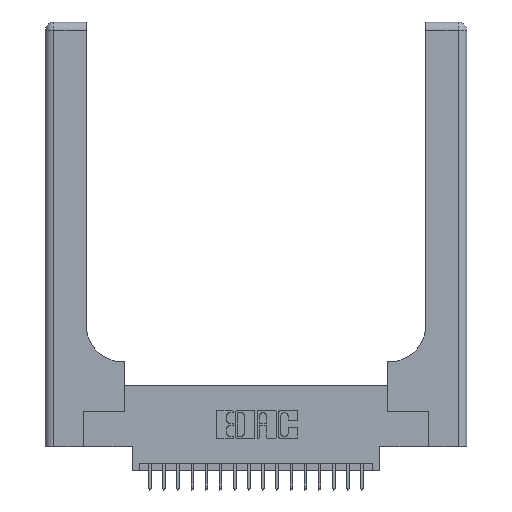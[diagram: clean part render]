
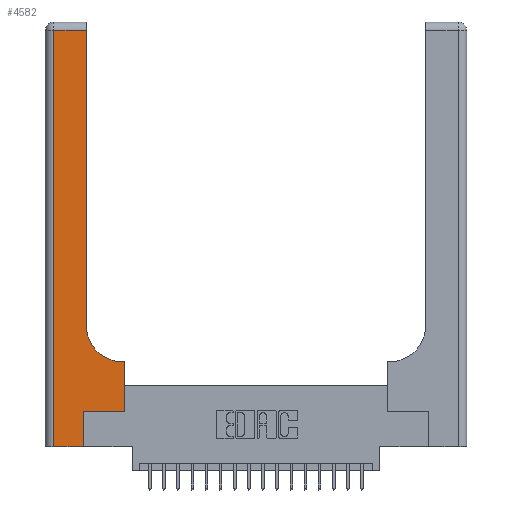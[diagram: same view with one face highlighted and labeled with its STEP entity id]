
A CAD part, top view. The second image highlights one B-rep face of the part: STEP entity #4582.
In plain terms, the highlighted planar face has unit normal (0, 0, 1).
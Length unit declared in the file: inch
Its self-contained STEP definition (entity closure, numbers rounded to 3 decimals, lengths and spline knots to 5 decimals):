
#65 = VECTOR ( 'NONE', #2025, 39.37008 ) ;
#373 = ORIENTED_EDGE ( 'NONE', *, *, #1104, .T. ) ;
#725 = LINE ( 'NONE', #10948, #19085 ) ;
#1032 = LINE ( 'NONE', #9504, #5738 ) ;
#1104 = EDGE_CURVE ( 'NONE', #9054, #12072, #725, .T. ) ;
#1222 = DIRECTION ( 'NONE',  ( 0., 1., 0. ) ) ;
#1312 = DIRECTION ( 'NONE',  ( 1., 0., 0. ) ) ;
#1569 = ORIENTED_EDGE ( 'NONE', *, *, #2822, .T. ) ;
#1586 = CARTESIAN_POINT ( 'NONE',  ( 0.2915, 0.85, 0.37 ) ) ;
#1832 = VECTOR ( 'NONE', #1312, 39.37008 ) ;
#2025 = DIRECTION ( 'NONE',  ( 0., 1., 0. ) ) ;
#2131 = CARTESIAN_POINT ( 'NONE',  ( 0.2915, 3., 0.37 ) ) ;
#2689 = ORIENTED_EDGE ( 'NONE', *, *, #15109, .T. ) ;
#2710 = ORIENTED_EDGE ( 'NONE', *, *, #3359, .T. ) ;
#2822 = EDGE_CURVE ( 'NONE', #18340, #11618, #16346, .T. ) ;
#2867 = LINE ( 'NONE', #9477, #3007 ) ;
#2895 = DIRECTION ( 'NONE',  ( 0., -1., 0. ) ) ;
#3000 = DIRECTION ( 'NONE',  ( -1., 0., 0. ) ) ;
#3007 = VECTOR ( 'NONE', #1222, 39.37008 ) ;
#3126 = PLANE ( 'NONE',  #5257 ) ;
#3159 = DIRECTION ( 'NONE',  ( 0., 0., -1. ) ) ;
#3212 = CARTESIAN_POINT ( 'NONE',  ( 0.2915, 0.6, 0.37 ) ) ;
#3359 = EDGE_CURVE ( 'NONE', #11618, #13096, #11821, .T. ) ;
#3872 = EDGE_CURVE ( 'NONE', #13096, #9054, #20190, .T. ) ;
#4400 = VECTOR ( 'NONE', #17076, 39.37008 ) ;
#4582 = ADVANCED_FACE ( 'NONE', ( #13520 ), #3126, .F. ) ;
#4727 = EDGE_LOOP ( 'NONE', ( #6545, #373, #9409, #11689, #12705, #2689, #13327, #1569, #2710 ) ) ;
#4884 = AXIS2_PLACEMENT_3D ( 'NONE', #16838, #3159, #9756 ) ;
#5224 = CARTESIAN_POINT ( 'NONE',  ( 0.5585, 0.25, 0.37 ) ) ;
#5257 = AXIS2_PLACEMENT_3D ( 'NONE', #11797, #18008, #20179 ) ;
#5450 = EDGE_CURVE ( 'NONE', #14862, #18210, #11525, .T. ) ;
#5738 = VECTOR ( 'NONE', #2895, 39.37008 ) ;
#6545 = ORIENTED_EDGE ( 'NONE', *, *, #3872, .T. ) ;
#7923 = CARTESIAN_POINT ( 'NONE',  ( 0.5585, 0.25, 0.37 ) ) ;
#8680 = VECTOR ( 'NONE', #3000, 39.37008 ) ;
#9054 = VERTEX_POINT ( 'NONE', #18430 ) ;
#9409 = ORIENTED_EDGE ( 'NONE', *, *, #19725, .T. ) ;
#9477 = CARTESIAN_POINT ( 'NONE',  ( 0.269, 0., 0.37 ) ) ;
#9504 = CARTESIAN_POINT ( 'NONE',  ( 0.06, 3., 0.37 ) ) ;
#9584 = DIRECTION ( 'NONE',  ( 1., 0., 0. ) ) ;
#9683 = LINE ( 'NONE', #14704, #11200 ) ;
#9756 = DIRECTION ( 'NONE',  ( 1., 0., 0. ) ) ;
#9996 = LINE ( 'NONE', #5224, #4400 ) ;
#10646 = CARTESIAN_POINT ( 'NONE',  ( 0.269, 0.25, 0.37 ) ) ;
#10948 = CARTESIAN_POINT ( 'NONE',  ( 0., 2.94, 0.37 ) ) ;
#11200 = VECTOR ( 'NONE', #9584, 39.37008 ) ;
#11525 = LINE ( 'NONE', #20033, #1832 ) ;
#11618 = VERTEX_POINT ( 'NONE', #14951 ) ;
#11689 = ORIENTED_EDGE ( 'NONE', *, *, #5450, .T. ) ;
#11797 = CARTESIAN_POINT ( 'NONE',  ( 0., 3., 0.37 ) ) ;
#11821 = CIRCLE ( 'NONE', #4884, 0.25 ) ;
#12072 = VERTEX_POINT ( 'NONE', #15541 ) ;
#12705 = ORIENTED_EDGE ( 'NONE', *, *, #20772, .T. ) ;
#12996 = CARTESIAN_POINT ( 'NONE',  ( 0.5585, 0.6, 0.37 ) ) ;
#13096 = VERTEX_POINT ( 'NONE', #1586 ) ;
#13327 = ORIENTED_EDGE ( 'NONE', *, *, #19140, .T. ) ;
#13520 = FACE_OUTER_BOUND ( 'NONE', #4727, .T. ) ;
#14704 = CARTESIAN_POINT ( 'NONE',  ( 0.269, 0.25, 0.37 ) ) ;
#14862 = VERTEX_POINT ( 'NONE', #18536 ) ;
#14951 = CARTESIAN_POINT ( 'NONE',  ( 0.5415, 0.6, 0.37 ) ) ;
#15109 = EDGE_CURVE ( 'NONE', #17607, #17696, #9683, .T. ) ;
#15541 = CARTESIAN_POINT ( 'NONE',  ( 0.06, 2.94, 0.37 ) ) ;
#16346 = LINE ( 'NONE', #3212, #8680 ) ;
#16838 = CARTESIAN_POINT ( 'NONE',  ( 0.5415, 0.85, 0.37 ) ) ;
#17076 = DIRECTION ( 'NONE',  ( 0., 1., 0. ) ) ;
#17607 = VERTEX_POINT ( 'NONE', #10646 ) ;
#17696 = VERTEX_POINT ( 'NONE', #7923 ) ;
#18008 = DIRECTION ( 'NONE',  ( 0., 0., -1. ) ) ;
#18210 = VERTEX_POINT ( 'NONE', #20861 ) ;
#18340 = VERTEX_POINT ( 'NONE', #12996 ) ;
#18430 = CARTESIAN_POINT ( 'NONE',  ( 0.2915, 2.94, 0.37 ) ) ;
#18536 = CARTESIAN_POINT ( 'NONE',  ( 0.06, 0., 0.37 ) ) ;
#19085 = VECTOR ( 'NONE', #21073, 39.37008 ) ;
#19140 = EDGE_CURVE ( 'NONE', #17696, #18340, #9996, .T. ) ;
#19725 = EDGE_CURVE ( 'NONE', #12072, #14862, #1032, .T. ) ;
#20033 = CARTESIAN_POINT ( 'NONE',  ( 0., 0., 0.37 ) ) ;
#20179 = DIRECTION ( 'NONE',  ( -1., 0., 0. ) ) ;
#20190 = LINE ( 'NONE', #2131, #65 ) ;
#20772 = EDGE_CURVE ( 'NONE', #18210, #17607, #2867, .T. ) ;
#20861 = CARTESIAN_POINT ( 'NONE',  ( 0.269, 0., 0.37 ) ) ;
#21073 = DIRECTION ( 'NONE',  ( -1., 0., 0. ) ) ;
